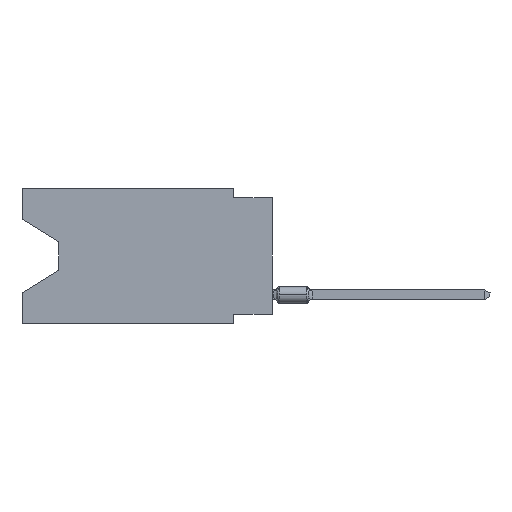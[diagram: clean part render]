
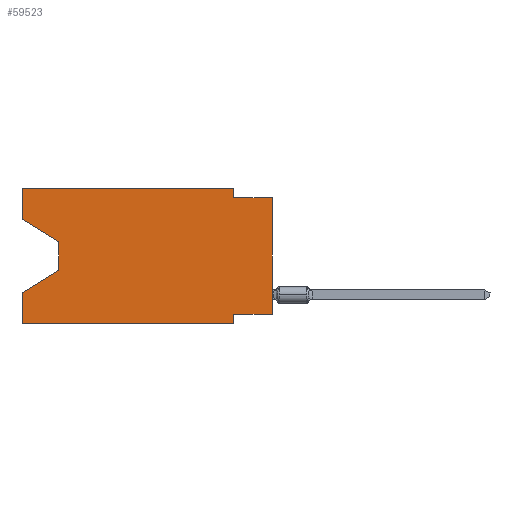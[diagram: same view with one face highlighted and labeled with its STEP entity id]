
A CAD part, left-side view. The second image highlights one B-rep face of the part: STEP entity #59523.
In plain terms, the highlighted planar face has unit normal (-1, 0, 0).
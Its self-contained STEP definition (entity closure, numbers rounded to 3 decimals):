
#91 = LINE ( 'NONE', #60026, #102 ) ;
#102 = VECTOR ( 'NONE', #29475, 1000. ) ;
#238 = VECTOR ( 'NONE', #68036, 1000. ) ;
#780 = VERTEX_POINT ( 'NONE', #39519 ) ;
#877 = VECTOR ( 'NONE', #26578, 1000. ) ;
#1206 = VECTOR ( 'NONE', #55857, 1000. ) ;
#1361 = LINE ( 'NONE', #38258, #9073 ) ;
#2230 = EDGE_CURVE ( 'NONE', #42534, #51355, #1361, .T. ) ;
#2538 = EDGE_CURVE ( 'NONE', #19134, #39291, #91, .T. ) ;
#3523 = EDGE_LOOP ( 'NONE', ( #38641, #69855, #18224, #72758, #31328, #42465, #77742, #64575, #67956, #53382, #50944, #48308 ) ) ;
#6276 = CARTESIAN_POINT ( 'NONE',  ( 0., 0., -0.635 ) ) ;
#6447 = LINE ( 'NONE', #74259, #75576 ) ;
#6459 = DIRECTION ( 'NONE',  ( 0., 0., -1. ) ) ;
#7275 = EDGE_CURVE ( 'NONE', #50039, #58836, #6447, .T. ) ;
#7454 = VERTEX_POINT ( 'NONE', #20694 ) ;
#9073 = VECTOR ( 'NONE', #31127, 1000. ) ;
#10985 = LINE ( 'NONE', #24086, #71363 ) ;
#13069 = EDGE_CURVE ( 'NONE', #780, #42534, #62497, .T. ) ;
#13786 = CARTESIAN_POINT ( 'NONE',  ( 0., 13.97, -3.505 ) ) ;
#13979 = EDGE_CURVE ( 'NONE', #59285, #58836, #51990, .T. ) ;
#14117 = DIRECTION ( 'NONE',  ( 0., 1., 0. ) ) ;
#14522 = EDGE_CURVE ( 'NONE', #50039, #39291, #10985, .T. ) ;
#14708 = LINE ( 'NONE', #44881, #68141 ) ;
#16906 = EDGE_CURVE ( 'NONE', #780, #7454, #50009, .T. ) ;
#17168 = CARTESIAN_POINT ( 'NONE',  ( 0., 2.54, -8.255 ) ) ;
#18224 = ORIENTED_EDGE ( 'NONE', *, *, #2538, .T. ) ;
#19134 = VERTEX_POINT ( 'NONE', #66427 ) ;
#20238 = CARTESIAN_POINT ( 'NONE',  ( 0., 16.383, -2.038 ) ) ;
#20694 = CARTESIAN_POINT ( 'NONE',  ( 0., 13.97, -3.505 ) ) ;
#20867 = LINE ( 'NONE', #63300, #56618 ) ;
#24086 = CARTESIAN_POINT ( 'NONE',  ( 0., 16.383, 0. ) ) ;
#24610 = CARTESIAN_POINT ( 'NONE',  ( 0., 16.383, -6.852 ) ) ;
#25477 = PLANE ( 'NONE',  #33963 ) ;
#26487 = LINE ( 'NONE', #13786, #1206 ) ;
#26578 = DIRECTION ( 'NONE',  ( 0., -0.855, -0.519 ) ) ;
#29475 = DIRECTION ( 'NONE',  ( 0., 0.855, -0.519 ) ) ;
#29866 = FACE_OUTER_BOUND ( 'NONE', #3523, .T. ) ;
#29981 = LINE ( 'NONE', #77966, #41828 ) ;
#31127 = DIRECTION ( 'NONE',  ( 0., -1., 0. ) ) ;
#31328 = ORIENTED_EDGE ( 'NONE', *, *, #7275, .T. ) ;
#32299 = LINE ( 'NONE', #67251, #238 ) ;
#32739 = DIRECTION ( 'NONE',  ( 0., 0., 1. ) ) ;
#33963 = AXIS2_PLACEMENT_3D ( 'NONE', #60798, #49286, #6459 ) ;
#35637 = CARTESIAN_POINT ( 'NONE',  ( 0., 16.383, 0. ) ) ;
#38258 = CARTESIAN_POINT ( 'NONE',  ( 0., 16.383, 0. ) ) ;
#38641 = ORIENTED_EDGE ( 'NONE', *, *, #16906, .T. ) ;
#39291 = VERTEX_POINT ( 'NONE', #24610 ) ;
#39519 = CARTESIAN_POINT ( 'NONE',  ( 0., 16.383, -2.038 ) ) ;
#41166 = EDGE_CURVE ( 'NONE', #7454, #19134, #26487, .T. ) ;
#41828 = VECTOR ( 'NONE', #70859, 1000. ) ;
#42465 = ORIENTED_EDGE ( 'NONE', *, *, #13979, .F. ) ;
#42534 = VERTEX_POINT ( 'NONE', #35637 ) ;
#44881 = CARTESIAN_POINT ( 'NONE',  ( 0., 0., -0.635 ) ) ;
#46029 = CARTESIAN_POINT ( 'NONE',  ( 0., 2.54, -8.89 ) ) ;
#47922 = CARTESIAN_POINT ( 'NONE',  ( 0., 16.383, -8.89 ) ) ;
#48308 = ORIENTED_EDGE ( 'NONE', *, *, #13069, .F. ) ;
#49286 = DIRECTION ( 'NONE',  ( 1., 0., 0. ) ) ;
#49488 = EDGE_CURVE ( 'NONE', #72905, #72722, #14708, .T. ) ;
#49896 = CARTESIAN_POINT ( 'NONE',  ( 0., 2.54, -0.635 ) ) ;
#50009 = LINE ( 'NONE', #20238, #877 ) ;
#50039 = VERTEX_POINT ( 'NONE', #47922 ) ;
#50944 = ORIENTED_EDGE ( 'NONE', *, *, #2230, .F. ) ;
#51355 = VERTEX_POINT ( 'NONE', #53050 ) ;
#51990 = LINE ( 'NONE', #46029, #75105 ) ;
#53050 = CARTESIAN_POINT ( 'NONE',  ( 0., 2.54, 0. ) ) ;
#53382 = ORIENTED_EDGE ( 'NONE', *, *, #64235, .F. ) ;
#55857 = DIRECTION ( 'NONE',  ( 0., 0., -1. ) ) ;
#56618 = VECTOR ( 'NONE', #14117, 1000. ) ;
#57178 = DIRECTION ( 'NONE',  ( 0., -1., 0. ) ) ;
#57342 = CARTESIAN_POINT ( 'NONE',  ( 0., 16.383, 0. ) ) ;
#57562 = EDGE_CURVE ( 'NONE', #73172, #59285, #20867, .T. ) ;
#58836 = VERTEX_POINT ( 'NONE', #68985 ) ;
#59285 = VERTEX_POINT ( 'NONE', #17168 ) ;
#59523 = ADVANCED_FACE ( 'NONE', ( #29866 ), #25477, .F. ) ;
#60026 = CARTESIAN_POINT ( 'NONE',  ( 0., 13.97, -5.385 ) ) ;
#60798 = CARTESIAN_POINT ( 'NONE',  ( 0., 16.383, 0. ) ) ;
#62296 = VECTOR ( 'NONE', #32739, 1000. ) ;
#62497 = LINE ( 'NONE', #57342, #62296 ) ;
#63300 = CARTESIAN_POINT ( 'NONE',  ( 0., 0., -8.255 ) ) ;
#63477 = DIRECTION ( 'NONE',  ( 0., 0., -1. ) ) ;
#64235 = EDGE_CURVE ( 'NONE', #51355, #72905, #32299, .T. ) ;
#64575 = ORIENTED_EDGE ( 'NONE', *, *, #71895, .T. ) ;
#66427 = CARTESIAN_POINT ( 'NONE',  ( 0., 13.97, -5.385 ) ) ;
#67251 = CARTESIAN_POINT ( 'NONE',  ( 0., 2.54, 0. ) ) ;
#67956 = ORIENTED_EDGE ( 'NONE', *, *, #49488, .F. ) ;
#68036 = DIRECTION ( 'NONE',  ( 0., 0., -1. ) ) ;
#68141 = VECTOR ( 'NONE', #57178, 1000. ) ;
#68985 = CARTESIAN_POINT ( 'NONE',  ( 0., 2.54, -8.89 ) ) ;
#69855 = ORIENTED_EDGE ( 'NONE', *, *, #41166, .T. ) ;
#70859 = DIRECTION ( 'NONE',  ( 0., 0., 1. ) ) ;
#71363 = VECTOR ( 'NONE', #77630, 1000. ) ;
#71658 = CARTESIAN_POINT ( 'NONE',  ( 0., 0., -8.255 ) ) ;
#71895 = EDGE_CURVE ( 'NONE', #73172, #72722, #29981, .T. ) ;
#72722 = VERTEX_POINT ( 'NONE', #6276 ) ;
#72758 = ORIENTED_EDGE ( 'NONE', *, *, #14522, .F. ) ;
#72905 = VERTEX_POINT ( 'NONE', #49896 ) ;
#73172 = VERTEX_POINT ( 'NONE', #71658 ) ;
#73474 = DIRECTION ( 'NONE',  ( 0., -1., 0. ) ) ;
#74259 = CARTESIAN_POINT ( 'NONE',  ( 0., 16.383, -8.89 ) ) ;
#75105 = VECTOR ( 'NONE', #63477, 1000. ) ;
#75576 = VECTOR ( 'NONE', #73474, 1000. ) ;
#77630 = DIRECTION ( 'NONE',  ( 0., 0., 1. ) ) ;
#77742 = ORIENTED_EDGE ( 'NONE', *, *, #57562, .F. ) ;
#77966 = CARTESIAN_POINT ( 'NONE',  ( 0., 0., 0. ) ) ;
